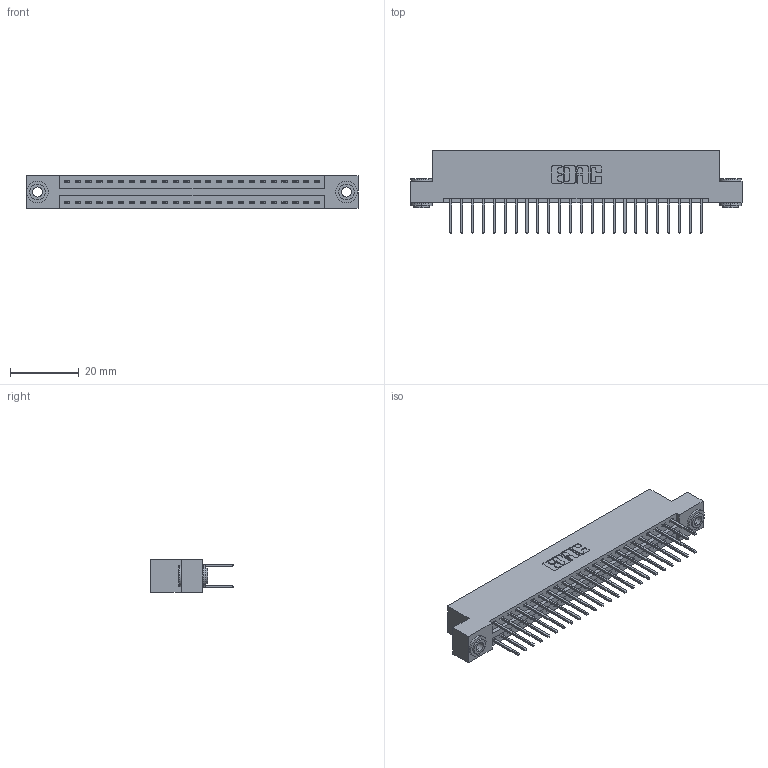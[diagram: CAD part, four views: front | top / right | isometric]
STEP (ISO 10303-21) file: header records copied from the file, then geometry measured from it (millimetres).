
FILE_DESCRIPTION (( 'STEP AP203' ), '1' );
FILE_NAME ('346-048-526-203.STEP', '2022-05-20T21:22:50', ( '' ), ( '' ), 'SwSTEP 2.0', 'SolidWorks 2020', '' );
FILE_SCHEMA (( 'CONFIG_CONTROL_DESIGN' ));
Length unit declared in the file: inch
Products named in the file (4): 345-250-002_345-250-002-102; 345-292-001_345-293-126; 346 Part_Flush Mounting Lugs - 0.156 Dia-TH; 346-048-526-203
Assembly tree (51 placements, depth 2):
  346-048-526-203
    346 Part_Flush Mounting Lugs - 0.156 Dia-TH
    345-292-001_345-293-126  x48
    345-250-002_345-250-002-102  x2
Bounding box: 96.77 x 24.13 x 9.4 mm (x, y, z)
Volume: 9376.9 mm3; surface area: 13207.3 mm2
Topology: 51 solids, 51 shells, 2670 faces, 7881 edges, 5186 vertices
Faces by surface type: plane 1780, cylinder 882, cone 8
Entity records: 19170 total; most frequent: CARTESIAN_POINT 3165, ORIENTED_EDGE 3090, DIRECTION 2871, EDGE_CURVE 1545, VECTOR 1293, LINE 1293, VERTEX_POINT 1026, AXIS2_PLACEMENT_3D 789
